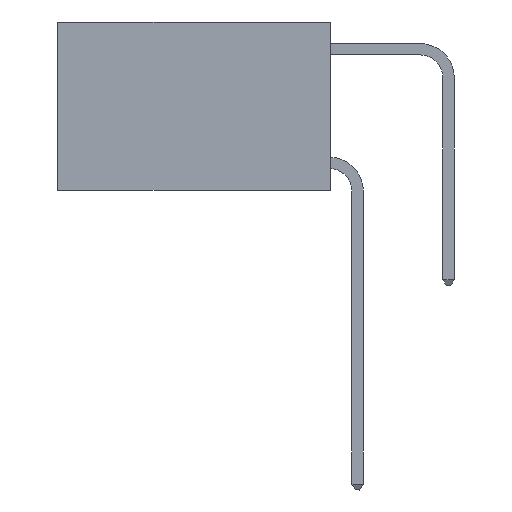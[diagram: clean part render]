
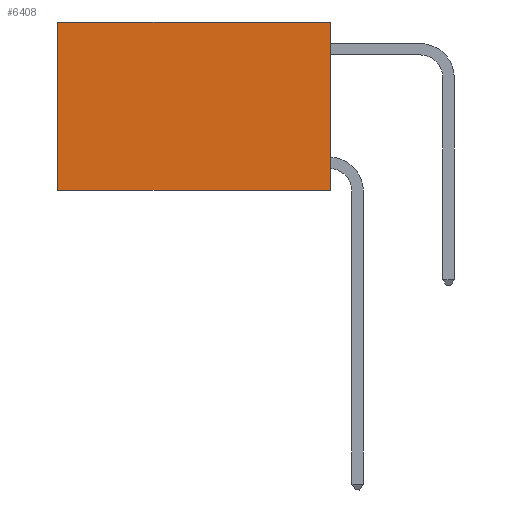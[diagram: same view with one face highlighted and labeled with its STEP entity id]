
A CAD part, left-side view. The second image highlights one B-rep face of the part: STEP entity #6408.
In plain terms, the highlighted planar face has unit normal (-1, 0, 0).
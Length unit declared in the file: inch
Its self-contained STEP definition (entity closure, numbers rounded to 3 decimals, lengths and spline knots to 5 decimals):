
#312 = DIRECTION ( 'NONE',  ( 0., 0., -1. ) ) ;
#334 = EDGE_CURVE ( 'NONE', #9237, #10424, #970, .T. ) ;
#756 = LINE ( 'NONE', #4669, #3104 ) ;
#809 = ORIENTED_EDGE ( 'NONE', *, *, #1268, .F. ) ;
#886 = VECTOR ( 'NONE', #9906, 39.37008 ) ;
#970 = LINE ( 'NONE', #3822, #886 ) ;
#1033 = CARTESIAN_POINT ( 'NONE',  ( 0.2625, 0., 0. ) ) ;
#1230 = CARTESIAN_POINT ( 'NONE',  ( 0.2625, 0.6, -0.37 ) ) ;
#1268 = EDGE_CURVE ( 'NONE', #9237, #4877, #756, .T. ) ;
#1321 = ORIENTED_EDGE ( 'NONE', *, *, #334, .T. ) ;
#2056 = PLANE ( 'NONE',  #6859 ) ;
#2622 = LINE ( 'NONE', #11915, #12228 ) ;
#2745 = ORIENTED_EDGE ( 'NONE', *, *, #7916, .T. ) ;
#3046 = DIRECTION ( 'NONE',  ( 0., 0., -1. ) ) ;
#3104 = VECTOR ( 'NONE', #4859, 39.37008 ) ;
#3413 = EDGE_LOOP ( 'NONE', ( #2745, #5601, #809, #1321 ) ) ;
#3822 = CARTESIAN_POINT ( 'NONE',  ( 0.2625, 0., 0. ) ) ;
#4009 = VERTEX_POINT ( 'NONE', #1230 ) ;
#4669 = CARTESIAN_POINT ( 'NONE',  ( 0.2625, 0., 0. ) ) ;
#4859 = DIRECTION ( 'NONE',  ( 0., 0., -1. ) ) ;
#4877 = VERTEX_POINT ( 'NONE', #11450 ) ;
#5298 = FACE_OUTER_BOUND ( 'NONE', #3413, .T. ) ;
#5601 = ORIENTED_EDGE ( 'NONE', *, *, #8233, .F. ) ;
#5806 = DIRECTION ( 'NONE',  ( 0., 1., 0. ) ) ;
#6408 = ADVANCED_FACE ( 'NONE', ( #5298 ), #2056, .F. ) ;
#6859 = AXIS2_PLACEMENT_3D ( 'NONE', #1033, #8869, #3046 ) ;
#7916 = EDGE_CURVE ( 'NONE', #10424, #4009, #2622, .T. ) ;
#8233 = EDGE_CURVE ( 'NONE', #4877, #4009, #8707, .T. ) ;
#8707 = LINE ( 'NONE', #12430, #10893 ) ;
#8869 = DIRECTION ( 'NONE',  ( 1., 0., 0. ) ) ;
#9237 = VERTEX_POINT ( 'NONE', #11897 ) ;
#9906 = DIRECTION ( 'NONE',  ( 0., 1., 0. ) ) ;
#10096 = CARTESIAN_POINT ( 'NONE',  ( 0.2625, 0.6, 0. ) ) ;
#10424 = VERTEX_POINT ( 'NONE', #10096 ) ;
#10893 = VECTOR ( 'NONE', #5806, 39.37008 ) ;
#11450 = CARTESIAN_POINT ( 'NONE',  ( 0.2625, 0., -0.37 ) ) ;
#11897 = CARTESIAN_POINT ( 'NONE',  ( 0.2625, 0., 0. ) ) ;
#11915 = CARTESIAN_POINT ( 'NONE',  ( 0.2625, 0.6, 0. ) ) ;
#12228 = VECTOR ( 'NONE', #312, 39.37008 ) ;
#12430 = CARTESIAN_POINT ( 'NONE',  ( 0.2625, 0., -0.37 ) ) ;
